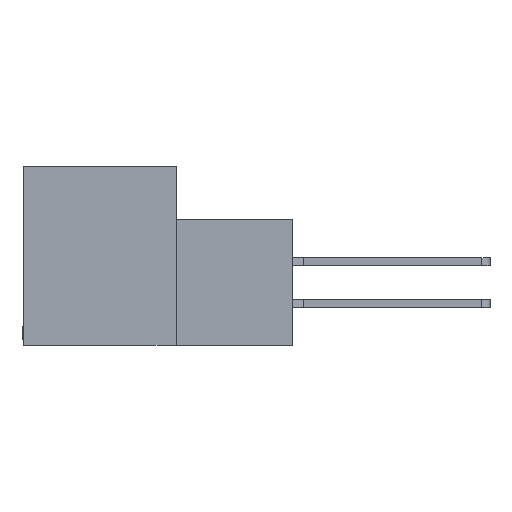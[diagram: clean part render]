
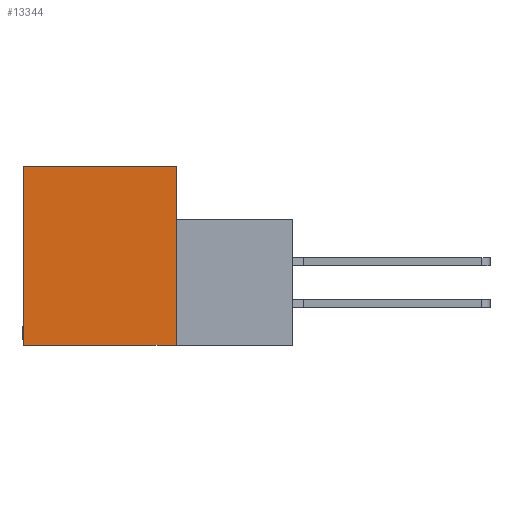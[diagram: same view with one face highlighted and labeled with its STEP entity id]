
A CAD part, left-side view. The second image highlights one B-rep face of the part: STEP entity #13344.
In plain terms, the highlighted planar face has unit normal (-1, 0, 0).
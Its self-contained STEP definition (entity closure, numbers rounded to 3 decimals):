
#28 = EDGE_CURVE ( 'NONE', #1237, #5355, #8078, .T. ) ;
#485 = CARTESIAN_POINT ( 'NONE',  ( 0., 0., 0. ) ) ;
#902 = DIRECTION ( 'NONE',  ( 0., -1., 0. ) ) ;
#1045 = CARTESIAN_POINT ( 'NONE',  ( 0., 11.506, -13.487 ) ) ;
#1237 = VERTEX_POINT ( 'NONE', #485 ) ;
#1446 = PLANE ( 'NONE',  #18778 ) ;
#1701 = LINE ( 'NONE', #21768, #18153 ) ;
#2138 = EDGE_CURVE ( 'NONE', #7416, #1237, #23297, .T. ) ;
#4884 = CARTESIAN_POINT ( 'NONE',  ( 0., 0., 0. ) ) ;
#5355 = VERTEX_POINT ( 'NONE', #12046 ) ;
#6571 = DIRECTION ( 'NONE',  ( 0., 0., -1. ) ) ;
#7416 = VERTEX_POINT ( 'NONE', #12173 ) ;
#7896 = ORIENTED_EDGE ( 'NONE', *, *, #13287, .F. ) ;
#8078 = LINE ( 'NONE', #4884, #10677 ) ;
#8333 = CARTESIAN_POINT ( 'NONE',  ( 0., -8.814, -13.487 ) ) ;
#9240 = ORIENTED_EDGE ( 'NONE', *, *, #21430, .F. ) ;
#10677 = VECTOR ( 'NONE', #6571, 1000. ) ;
#11195 = VECTOR ( 'NONE', #12045, 1000. ) ;
#11929 = CARTESIAN_POINT ( 'NONE',  ( 0., 11.506, 0. ) ) ;
#12045 = DIRECTION ( 'NONE',  ( 0., 1., 0. ) ) ;
#12046 = CARTESIAN_POINT ( 'NONE',  ( 0., 0., -13.487 ) ) ;
#12173 = CARTESIAN_POINT ( 'NONE',  ( 0., 11.506, 0. ) ) ;
#13113 = ORIENTED_EDGE ( 'NONE', *, *, #2138, .F. ) ;
#13287 = EDGE_CURVE ( 'NONE', #15366, #7416, #1701, .T. ) ;
#13344 = ADVANCED_FACE ( 'NONE', ( #23634 ), #1446, .F. ) ;
#14084 = CARTESIAN_POINT ( 'NONE',  ( 0., 0., 0. ) ) ;
#14379 = LINE ( 'NONE', #8333, #11195 ) ;
#15366 = VERTEX_POINT ( 'NONE', #1045 ) ;
#18153 = VECTOR ( 'NONE', #19908, 1000. ) ;
#18778 = AXIS2_PLACEMENT_3D ( 'NONE', #14084, #19665, #23840 ) ;
#18967 = ORIENTED_EDGE ( 'NONE', *, *, #28, .F. ) ;
#19665 = DIRECTION ( 'NONE',  ( 1., 0., 0. ) ) ;
#19908 = DIRECTION ( 'NONE',  ( 0., 0., 1. ) ) ;
#20139 = VECTOR ( 'NONE', #902, 1000. ) ;
#21430 = EDGE_CURVE ( 'NONE', #5355, #15366, #14379, .T. ) ;
#21768 = CARTESIAN_POINT ( 'NONE',  ( 0., 11.506, -13.487 ) ) ;
#23297 = LINE ( 'NONE', #11929, #20139 ) ;
#23405 = EDGE_LOOP ( 'NONE', ( #9240, #18967, #13113, #7896 ) ) ;
#23634 = FACE_OUTER_BOUND ( 'NONE', #23405, .T. ) ;
#23840 = DIRECTION ( 'NONE',  ( 0., 0., -1. ) ) ;
